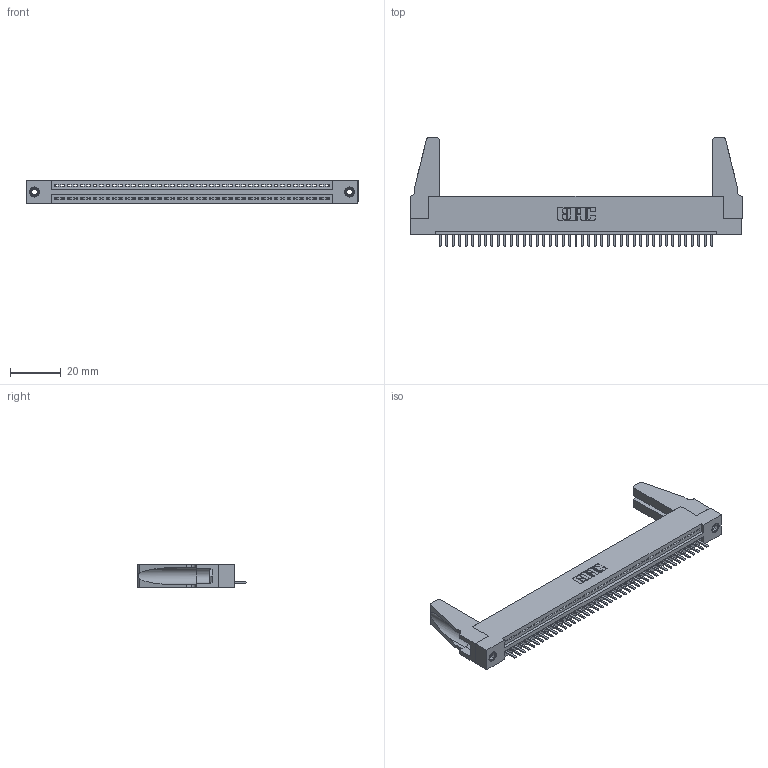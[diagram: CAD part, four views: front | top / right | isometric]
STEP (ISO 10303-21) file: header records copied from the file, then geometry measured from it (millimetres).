
FILE_DESCRIPTION (( 'STEP AP203' ), '1' );
FILE_NAME ('345-043-520-188.STEP', '2019-10-08T15:49:19', ( '' ), ( '' ), 'SwSTEP 2.0', 'SolidWorks 2016', '' );
FILE_SCHEMA (( 'CONFIG_CONTROL_DESIGN' ));
Length unit declared in the file: inch
Products named in the file (5): 345-250-001_345-250-001-102; 345-292-001_345-293-120; 345 Part_Flush Mounting Lugs - 0.156 Dia-TH; 345-043-520-188; 345-220-078_345-220-088
Assembly tree (48 placements, depth 2):
  345-043-520-188
    345 Part_Flush Mounting Lugs - 0.156 Dia-TH
    345-292-001_345-293-120  x43
    345-250-001_345-250-001-102  x2
    345-220-078_345-220-088  x2
Bounding box: 130.45 x 42.55 x 9.4 mm (x, y, z)
Volume: 15527.7 mm3; surface area: 19050.8 mm2
Topology: 48 solids, 48 shells, 2916 faces, 8567 edges, 5586 vertices
Faces by surface type: plane 1958, cylinder 942, cone 12, torus 4
Entity records: 34490 total; most frequent: CARTESIAN_POINT 5975, ORIENTED_EDGE 5900, DIRECTION 5212, EDGE_CURVE 2950, VECTOR 2600, LINE 2600, VERTEX_POINT 1958, AXIS2_PLACEMENT_3D 1306
